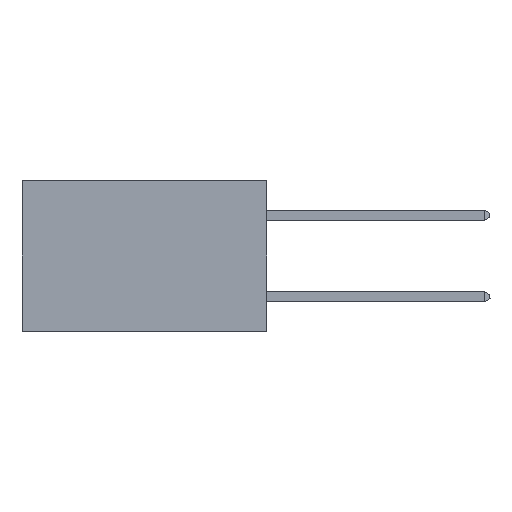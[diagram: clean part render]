
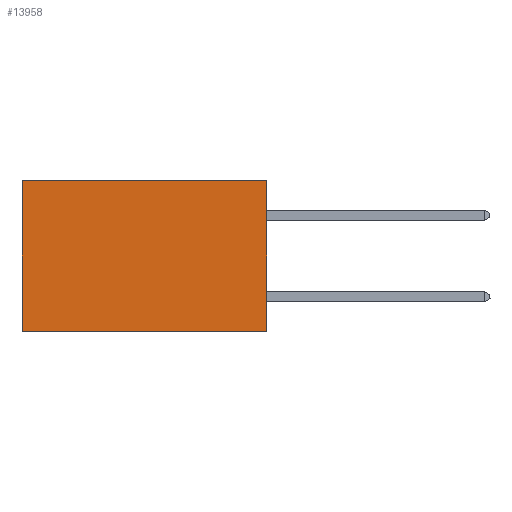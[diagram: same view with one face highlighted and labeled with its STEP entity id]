
A CAD part, left-side view. The second image highlights one B-rep face of the part: STEP entity #13958.
In plain terms, the highlighted planar face has unit normal (-1, 0, 0).
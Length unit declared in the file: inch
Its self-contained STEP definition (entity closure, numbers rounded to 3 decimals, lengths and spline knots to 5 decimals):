
#3377 = VECTOR ( 'NONE', #22659, 39.37008 ) ;
#4809 = DIRECTION ( 'NONE',  ( 0., 0., -1. ) ) ;
#5190 = AXIS2_PLACEMENT_3D ( 'NONE', #25759, #12951, #8954 ) ;
#5753 = DIRECTION ( 'NONE',  ( 0., 1., 0. ) ) ;
#6047 = ORIENTED_EDGE ( 'NONE', *, *, #17946, .F. ) ;
#6990 = FACE_OUTER_BOUND ( 'NONE', #21303, .T. ) ;
#7253 = EDGE_CURVE ( 'NONE', #18684, #22300, #15960, .T. ) ;
#8954 = DIRECTION ( 'NONE',  ( 0., 0., -1. ) ) ;
#10759 = PLANE ( 'NONE',  #5190 ) ;
#12875 = VERTEX_POINT ( 'NONE', #24486 ) ;
#12951 = DIRECTION ( 'NONE',  ( 1., 0., 0. ) ) ;
#13847 = CARTESIAN_POINT ( 'NONE',  ( 0.2875, 0., 0. ) ) ;
#13958 = ADVANCED_FACE ( 'NONE', ( #6990 ), #10759, .F. ) ;
#14217 = DIRECTION ( 'NONE',  ( 0., 1., 0. ) ) ;
#15521 = ORIENTED_EDGE ( 'NONE', *, *, #7253, .T. ) ;
#15960 = LINE ( 'NONE', #13847, #22686 ) ;
#17158 = CARTESIAN_POINT ( 'NONE',  ( 0.2875, 0., 0. ) ) ;
#17791 = LINE ( 'NONE', #18232, #3377 ) ;
#17822 = EDGE_CURVE ( 'NONE', #18684, #26903, #17791, .T. ) ;
#17946 = EDGE_CURVE ( 'NONE', #26903, #12875, #27529, .T. ) ;
#18232 = CARTESIAN_POINT ( 'NONE',  ( 0.2875, 0., 0. ) ) ;
#18604 = CARTESIAN_POINT ( 'NONE',  ( 0.2875, 0., -0.37 ) ) ;
#18684 = VERTEX_POINT ( 'NONE', #17158 ) ;
#19120 = CARTESIAN_POINT ( 'NONE',  ( 0.2875, 0.6, 0. ) ) ;
#19408 = EDGE_CURVE ( 'NONE', #22300, #12875, #25764, .T. ) ;
#19801 = CARTESIAN_POINT ( 'NONE',  ( 0.2875, 0.6, 0. ) ) ;
#20551 = CARTESIAN_POINT ( 'NONE',  ( 0.2875, 0., -0.37 ) ) ;
#21303 = EDGE_LOOP ( 'NONE', ( #27376, #6047, #24903, #15521 ) ) ;
#22300 = VERTEX_POINT ( 'NONE', #19120 ) ;
#22659 = DIRECTION ( 'NONE',  ( 0., 0., -1. ) ) ;
#22686 = VECTOR ( 'NONE', #14217, 39.37008 ) ;
#23218 = VECTOR ( 'NONE', #5753, 39.37008 ) ;
#24486 = CARTESIAN_POINT ( 'NONE',  ( 0.2875, 0.6, -0.37 ) ) ;
#24903 = ORIENTED_EDGE ( 'NONE', *, *, #17822, .F. ) ;
#25759 = CARTESIAN_POINT ( 'NONE',  ( 0.2875, 0., 0. ) ) ;
#25764 = LINE ( 'NONE', #19801, #26728 ) ;
#26728 = VECTOR ( 'NONE', #4809, 39.37008 ) ;
#26903 = VERTEX_POINT ( 'NONE', #20551 ) ;
#27376 = ORIENTED_EDGE ( 'NONE', *, *, #19408, .T. ) ;
#27529 = LINE ( 'NONE', #18604, #23218 ) ;
